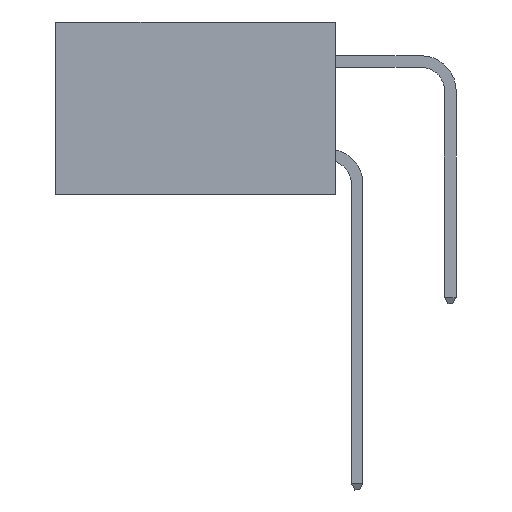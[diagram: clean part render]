
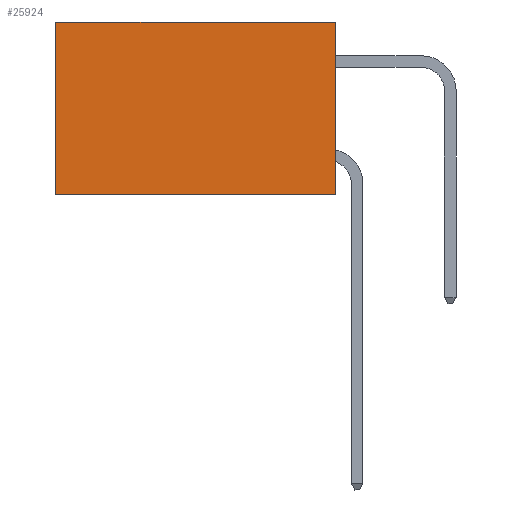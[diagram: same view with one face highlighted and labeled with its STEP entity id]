
A CAD part, left-side view. The second image highlights one B-rep face of the part: STEP entity #25924.
In plain terms, the highlighted planar face has unit normal (-1, 0, 0).
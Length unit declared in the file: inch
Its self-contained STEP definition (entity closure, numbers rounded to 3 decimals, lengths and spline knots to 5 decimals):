
#1872 = VERTEX_POINT ( 'NONE', #10721 ) ;
#1927 = CARTESIAN_POINT ( 'NONE',  ( 0.2875, 0.6, 0. ) ) ;
#2203 = CARTESIAN_POINT ( 'NONE',  ( 0.2875, 0., 0. ) ) ;
#2674 = FACE_OUTER_BOUND ( 'NONE', #20678, .T. ) ;
#3413 = VECTOR ( 'NONE', #29761, 39.37008 ) ;
#5616 = CARTESIAN_POINT ( 'NONE',  ( 0.2875, 0., 0. ) ) ;
#7450 = EDGE_CURVE ( 'NONE', #13570, #8857, #14800, .T. ) ;
#7667 = CARTESIAN_POINT ( 'NONE',  ( 0.2875, 0.6, 0. ) ) ;
#8849 = ORIENTED_EDGE ( 'NONE', *, *, #9622, .F. ) ;
#8857 = VERTEX_POINT ( 'NONE', #1927 ) ;
#9031 = CARTESIAN_POINT ( 'NONE',  ( 0.2875, 0., -0.37 ) ) ;
#9622 = EDGE_CURVE ( 'NONE', #27272, #1872, #22153, .T. ) ;
#10721 = CARTESIAN_POINT ( 'NONE',  ( 0.2875, 0.6, -0.37 ) ) ;
#11456 = EDGE_CURVE ( 'NONE', #13570, #27272, #13194, .T. ) ;
#11495 = VECTOR ( 'NONE', #27989, 39.37008 ) ;
#11532 = CARTESIAN_POINT ( 'NONE',  ( 0.2875, 0., -0.37 ) ) ;
#12588 = DIRECTION ( 'NONE',  ( 0., 0., -1. ) ) ;
#13194 = LINE ( 'NONE', #5616, #24980 ) ;
#13570 = VERTEX_POINT ( 'NONE', #23017 ) ;
#14125 = DIRECTION ( 'NONE',  ( 0., 0., -1. ) ) ;
#14800 = LINE ( 'NONE', #2203, #11495 ) ;
#18472 = PLANE ( 'NONE',  #26343 ) ;
#20678 = EDGE_LOOP ( 'NONE', ( #21269, #8849, #23067, #27015 ) ) ;
#21269 = ORIENTED_EDGE ( 'NONE', *, *, #28570, .T. ) ;
#22153 = LINE ( 'NONE', #9031, #3413 ) ;
#23017 = CARTESIAN_POINT ( 'NONE',  ( 0.2875, 0., 0. ) ) ;
#23067 = ORIENTED_EDGE ( 'NONE', *, *, #11456, .F. ) ;
#23877 = VECTOR ( 'NONE', #14125, 39.37008 ) ;
#24980 = VECTOR ( 'NONE', #26912, 39.37008 ) ;
#25924 = ADVANCED_FACE ( 'NONE', ( #2674 ), #18472, .F. ) ;
#26343 = AXIS2_PLACEMENT_3D ( 'NONE', #28844, #26616, #12588 ) ;
#26616 = DIRECTION ( 'NONE',  ( 1., 0., 0. ) ) ;
#26912 = DIRECTION ( 'NONE',  ( 0., 0., -1. ) ) ;
#27015 = ORIENTED_EDGE ( 'NONE', *, *, #7450, .T. ) ;
#27272 = VERTEX_POINT ( 'NONE', #11532 ) ;
#27989 = DIRECTION ( 'NONE',  ( 0., 1., 0. ) ) ;
#28570 = EDGE_CURVE ( 'NONE', #8857, #1872, #30116, .T. ) ;
#28844 = CARTESIAN_POINT ( 'NONE',  ( 0.2875, 0., 0. ) ) ;
#29761 = DIRECTION ( 'NONE',  ( 0., 1., 0. ) ) ;
#30116 = LINE ( 'NONE', #7667, #23877 ) ;
